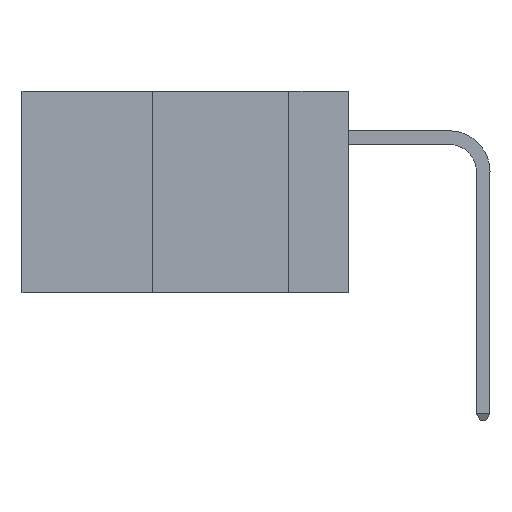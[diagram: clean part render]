
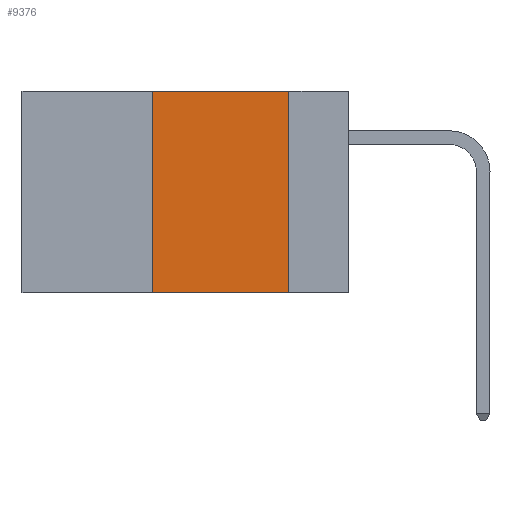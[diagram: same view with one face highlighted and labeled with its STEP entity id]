
A CAD part, left-side view. The second image highlights one B-rep face of the part: STEP entity #9376.
In plain terms, the highlighted planar face has unit normal (-1, 0, 0).
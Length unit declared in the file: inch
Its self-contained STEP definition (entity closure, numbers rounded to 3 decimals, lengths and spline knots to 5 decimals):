
#904 = VECTOR ( 'NONE', #8717, 39.37008 ) ;
#1723 = CARTESIAN_POINT ( 'NONE',  ( 0., 0.11, 0. ) ) ;
#3418 = ORIENTED_EDGE ( 'NONE', *, *, #7026, .F. ) ;
#3500 = EDGE_CURVE ( 'NONE', #27378, #6751, #23817, .T. ) ;
#4029 = CARTESIAN_POINT ( 'NONE',  ( 0., 0.6, 0. ) ) ;
#5856 = VECTOR ( 'NONE', #30396, 39.37008 ) ;
#6751 = VERTEX_POINT ( 'NONE', #7527 ) ;
#7026 = EDGE_CURVE ( 'NONE', #27378, #25667, #9568, .T. ) ;
#7527 = CARTESIAN_POINT ( 'NONE',  ( 0., 0.11, -0.37 ) ) ;
#8614 = DIRECTION ( 'NONE',  ( 0., 0., -1. ) ) ;
#8717 = DIRECTION ( 'NONE',  ( 0., -1., 0. ) ) ;
#9376 = ADVANCED_FACE ( 'NONE', ( #16098 ), #20862, .F. ) ;
#9568 = LINE ( 'NONE', #16682, #5856 ) ;
#11025 = CARTESIAN_POINT ( 'NONE',  ( 0., 0.6, -0.37 ) ) ;
#14347 = CARTESIAN_POINT ( 'NONE',  ( 0., 0.36, 0. ) ) ;
#14983 = EDGE_LOOP ( 'NONE', ( #30230, #17021, #3418, #22163 ) ) ;
#15332 = DIRECTION ( 'NONE',  ( 0., -1., 0. ) ) ;
#15705 = DIRECTION ( 'NONE',  ( 0., 0., -1. ) ) ;
#15817 = DIRECTION ( 'NONE',  ( 1., 0., 0. ) ) ;
#15906 = VERTEX_POINT ( 'NONE', #23299 ) ;
#16098 = FACE_OUTER_BOUND ( 'NONE', #14983, .T. ) ;
#16682 = CARTESIAN_POINT ( 'NONE',  ( 0., 0.36, 0. ) ) ;
#17021 = ORIENTED_EDGE ( 'NONE', *, *, #24600, .F. ) ;
#19346 = VECTOR ( 'NONE', #8614, 39.37008 ) ;
#19764 = AXIS2_PLACEMENT_3D ( 'NONE', #4029, #15817, #15705 ) ;
#20356 = LINE ( 'NONE', #24727, #24821 ) ;
#20862 = PLANE ( 'NONE',  #19764 ) ;
#21362 = CARTESIAN_POINT ( 'NONE',  ( 0., 0.36, -0.37 ) ) ;
#22163 = ORIENTED_EDGE ( 'NONE', *, *, #3500, .T. ) ;
#23036 = EDGE_CURVE ( 'NONE', #15906, #6751, #25614, .T. ) ;
#23299 = CARTESIAN_POINT ( 'NONE',  ( 0., 0.11, 0. ) ) ;
#23817 = LINE ( 'NONE', #11025, #904 ) ;
#24600 = EDGE_CURVE ( 'NONE', #25667, #15906, #20356, .T. ) ;
#24727 = CARTESIAN_POINT ( 'NONE',  ( 0., 0.6, 0. ) ) ;
#24821 = VECTOR ( 'NONE', #15332, 39.37008 ) ;
#25614 = LINE ( 'NONE', #1723, #19346 ) ;
#25667 = VERTEX_POINT ( 'NONE', #14347 ) ;
#27378 = VERTEX_POINT ( 'NONE', #21362 ) ;
#30230 = ORIENTED_EDGE ( 'NONE', *, *, #23036, .F. ) ;
#30396 = DIRECTION ( 'NONE',  ( 0., 0., 1. ) ) ;
